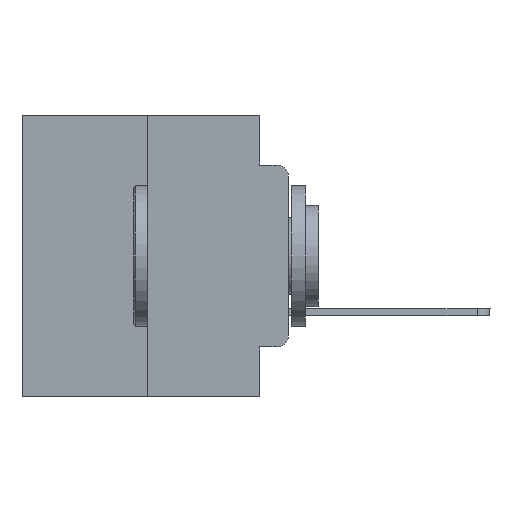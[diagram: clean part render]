
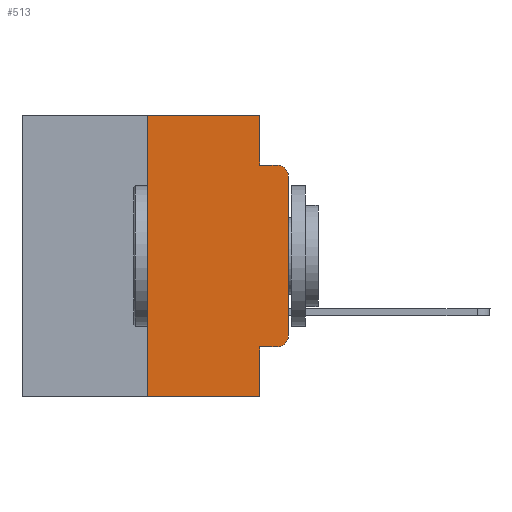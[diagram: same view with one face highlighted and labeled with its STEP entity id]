
A CAD part, left-side view. The second image highlights one B-rep face of the part: STEP entity #513.
In plain terms, the highlighted planar face has unit normal (-1, 0, 0).
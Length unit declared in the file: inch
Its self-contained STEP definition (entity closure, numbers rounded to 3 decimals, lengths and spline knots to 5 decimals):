
#23 = AXIS2_PLACEMENT_3D ( 'NONE', #4371, #25907, #23859 ) ;
#311 = FACE_OUTER_BOUND ( 'NONE', #12147, .T. ) ;
#321 = ORIENTED_EDGE ( 'NONE', *, *, #22152, .T. ) ;
#450 = ORIENTED_EDGE ( 'NONE', *, *, #24641, .T. ) ;
#513 = ADVANCED_FACE ( 'NONE', ( #311 ), #8896, .F. ) ;
#641 = EDGE_CURVE ( 'NONE', #8510, #17071, #17941, .T. ) ;
#680 = ORIENTED_EDGE ( 'NONE', *, *, #16337, .F. ) ;
#1501 = ORIENTED_EDGE ( 'NONE', *, *, #15925, .F. ) ;
#3323 = CARTESIAN_POINT ( 'NONE',  ( 0., 0.02, -0.1085 ) ) ;
#3425 = VERTEX_POINT ( 'NONE', #22033 ) ;
#3660 = CARTESIAN_POINT ( 'NONE',  ( 0., 0.02, -0.0885 ) ) ;
#3980 = AXIS2_PLACEMENT_3D ( 'NONE', #3323, #20171, #17937 ) ;
#4371 = CARTESIAN_POINT ( 'NONE',  ( 0., 0.473, 0. ) ) ;
#4665 = VERTEX_POINT ( 'NONE', #3660 ) ;
#4739 = VECTOR ( 'NONE', #26522, 39.37008 ) ;
#5111 = CARTESIAN_POINT ( 'NONE',  ( 0., 0.051, 0. ) ) ;
#6418 = VECTOR ( 'NONE', #24118, 39.37008 ) ;
#6816 = VERTEX_POINT ( 'NONE', #26323 ) ;
#7235 = VECTOR ( 'NONE', #17023, 39.37008 ) ;
#7714 = VECTOR ( 'NONE', #14215, 39.37008 ) ;
#7942 = VECTOR ( 'NONE', #26096, 39.37008 ) ;
#8050 = VECTOR ( 'NONE', #16669, 39.37008 ) ;
#8463 = CARTESIAN_POINT ( 'NONE',  ( 0., 0.02, -0.4115 ) ) ;
#8510 = VERTEX_POINT ( 'NONE', #15602 ) ;
#8896 = PLANE ( 'NONE',  #23 ) ;
#9348 = CARTESIAN_POINT ( 'NONE',  ( 0., 0.25, 0. ) ) ;
#9538 = CARTESIAN_POINT ( 'NONE',  ( 0., 0., 0. ) ) ;
#9733 = CARTESIAN_POINT ( 'NONE',  ( 0., 0.051, -0.0885 ) ) ;
#10517 = CARTESIAN_POINT ( 'NONE',  ( 0., 0.473, -0.5 ) ) ;
#11153 = VECTOR ( 'NONE', #20157, 39.37008 ) ;
#11858 = LINE ( 'NONE', #12021, #15836 ) ;
#12021 = CARTESIAN_POINT ( 'NONE',  ( 0., 0.051, -0.4115 ) ) ;
#12120 = DIRECTION ( 'NONE',  ( 0., 0., -1. ) ) ;
#12147 = EDGE_LOOP ( 'NONE', ( #321, #450, #24221, #680, #19526, #1501, #14932, #25364, #18476, #22310 ) ) ;
#12210 = DIRECTION ( 'NONE',  ( -1., 0., 0. ) ) ;
#13739 = LINE ( 'NONE', #26920, #8050 ) ;
#13743 = LINE ( 'NONE', #18393, #4739 ) ;
#14097 = VERTEX_POINT ( 'NONE', #8463 ) ;
#14215 = DIRECTION ( 'NONE',  ( 0., 0., -1. ) ) ;
#14932 = ORIENTED_EDGE ( 'NONE', *, *, #19114, .T. ) ;
#15006 = CARTESIAN_POINT ( 'NONE',  ( 0., 0.051, -0.5 ) ) ;
#15040 = AXIS2_PLACEMENT_3D ( 'NONE', #18694, #12210, #12120 ) ;
#15429 = LINE ( 'NONE', #16642, #7714 ) ;
#15602 = CARTESIAN_POINT ( 'NONE',  ( 0., 0.051, -0.4115 ) ) ;
#15836 = VECTOR ( 'NONE', #16395, 39.37008 ) ;
#15925 = EDGE_CURVE ( 'NONE', #3425, #26384, #23045, .T. ) ;
#16337 = EDGE_CURVE ( 'NONE', #21663, #22378, #15429, .T. ) ;
#16395 = DIRECTION ( 'NONE',  ( 0., -1., 0. ) ) ;
#16642 = CARTESIAN_POINT ( 'NONE',  ( 0., 0.051, 0. ) ) ;
#16669 = DIRECTION ( 'NONE',  ( 0., -1., 0. ) ) ;
#17023 = DIRECTION ( 'NONE',  ( 0., -1., 0. ) ) ;
#17071 = VERTEX_POINT ( 'NONE', #15006 ) ;
#17543 = CARTESIAN_POINT ( 'NONE',  ( 0., 0., -0.1085 ) ) ;
#17937 = DIRECTION ( 'NONE',  ( 0., 0., -1. ) ) ;
#17941 = LINE ( 'NONE', #5111, #7942 ) ;
#18393 = CARTESIAN_POINT ( 'NONE',  ( 0., 0.051, -0.0885 ) ) ;
#18476 = ORIENTED_EDGE ( 'NONE', *, *, #20869, .T. ) ;
#18694 = CARTESIAN_POINT ( 'NONE',  ( 0., 0.02, -0.3915 ) ) ;
#19114 = EDGE_CURVE ( 'NONE', #3425, #17071, #26514, .T. ) ;
#19526 = ORIENTED_EDGE ( 'NONE', *, *, #23553, .F. ) ;
#19768 = LINE ( 'NONE', #9538, #11153 ) ;
#19891 = CARTESIAN_POINT ( 'NONE',  ( 0., 0.051, 0. ) ) ;
#20157 = DIRECTION ( 'NONE',  ( 0., 0., 1. ) ) ;
#20171 = DIRECTION ( 'NONE',  ( -1., 0., 0. ) ) ;
#20672 = CIRCLE ( 'NONE', #3980, 0.02 ) ;
#20869 = EDGE_CURVE ( 'NONE', #8510, #14097, #11858, .T. ) ;
#21663 = VERTEX_POINT ( 'NONE', #19891 ) ;
#22033 = CARTESIAN_POINT ( 'NONE',  ( 0., 0.25, -0.5 ) ) ;
#22152 = EDGE_CURVE ( 'NONE', #6816, #22682, #19768, .T. ) ;
#22310 = ORIENTED_EDGE ( 'NONE', *, *, #23605, .T. ) ;
#22378 = VERTEX_POINT ( 'NONE', #9733 ) ;
#22682 = VERTEX_POINT ( 'NONE', #17543 ) ;
#23045 = LINE ( 'NONE', #9348, #6418 ) ;
#23553 = EDGE_CURVE ( 'NONE', #26384, #21663, #13739, .T. ) ;
#23605 = EDGE_CURVE ( 'NONE', #14097, #6816, #27321, .T. ) ;
#23859 = DIRECTION ( 'NONE',  ( 0., 0., -1. ) ) ;
#24118 = DIRECTION ( 'NONE',  ( 0., 0., 1. ) ) ;
#24129 = EDGE_CURVE ( 'NONE', #22378, #4665, #13743, .T. ) ;
#24221 = ORIENTED_EDGE ( 'NONE', *, *, #24129, .F. ) ;
#24641 = EDGE_CURVE ( 'NONE', #22682, #4665, #20672, .T. ) ;
#25364 = ORIENTED_EDGE ( 'NONE', *, *, #641, .F. ) ;
#25907 = DIRECTION ( 'NONE',  ( 1., 0., 0. ) ) ;
#26096 = DIRECTION ( 'NONE',  ( 0., 0., -1. ) ) ;
#26323 = CARTESIAN_POINT ( 'NONE',  ( 0., 0., -0.3915 ) ) ;
#26384 = VERTEX_POINT ( 'NONE', #26829 ) ;
#26514 = LINE ( 'NONE', #10517, #7235 ) ;
#26522 = DIRECTION ( 'NONE',  ( 0., -1., 0. ) ) ;
#26829 = CARTESIAN_POINT ( 'NONE',  ( 0., 0.25, 0. ) ) ;
#26920 = CARTESIAN_POINT ( 'NONE',  ( 0., 0.473, 0. ) ) ;
#27321 = CIRCLE ( 'NONE', #15040, 0.02 ) ;
